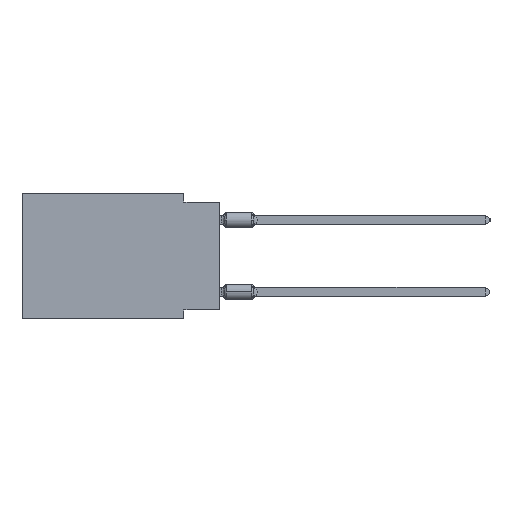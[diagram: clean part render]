
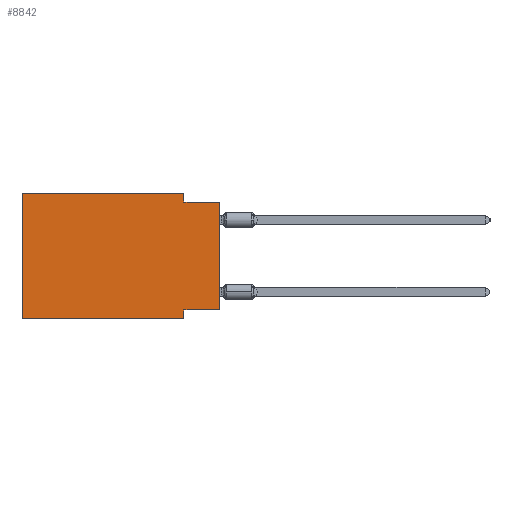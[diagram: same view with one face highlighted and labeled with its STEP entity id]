
A CAD part, left-side view. The second image highlights one B-rep face of the part: STEP entity #8842.
In plain terms, the highlighted planar face has unit normal (-1, 0, 0).
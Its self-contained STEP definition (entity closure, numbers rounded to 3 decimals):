
#359 = CARTESIAN_POINT ( 'NONE',  ( 0., 2.54, -8.89 ) ) ;
#743 = ORIENTED_EDGE ( 'NONE', *, *, #14845, .T. ) ;
#1000 = EDGE_CURVE ( 'NONE', #20234, #16087, #9139, .T. ) ;
#1103 = VECTOR ( 'NONE', #6230, 1000. ) ;
#1387 = EDGE_CURVE ( 'NONE', #20954, #15515, #6938, .T. ) ;
#1452 = DIRECTION ( 'NONE',  ( 0., -1., 0. ) ) ;
#2426 = CARTESIAN_POINT ( 'NONE',  ( 0., 13.97, -8.89 ) ) ;
#2891 = DIRECTION ( 'NONE',  ( 0., -1., 0. ) ) ;
#3227 = LINE ( 'NONE', #7388, #23684 ) ;
#3549 = CARTESIAN_POINT ( 'NONE',  ( 0., 0., -8.255 ) ) ;
#3810 = CARTESIAN_POINT ( 'NONE',  ( 0., 13.97, -8.89 ) ) ;
#3940 = CARTESIAN_POINT ( 'NONE',  ( 0., 13.97, 0. ) ) ;
#4109 = AXIS2_PLACEMENT_3D ( 'NONE', #7178, #11106, #23124 ) ;
#4303 = EDGE_LOOP ( 'NONE', ( #743, #24543, #21683, #19133, #11084, #18147, #22520, #16724 ) ) ;
#4856 = VECTOR ( 'NONE', #24507, 1000. ) ;
#5414 = CARTESIAN_POINT ( 'NONE',  ( 0., 2.54, -0.635 ) ) ;
#6230 = DIRECTION ( 'NONE',  ( 0., 0., -1. ) ) ;
#6813 = EDGE_CURVE ( 'NONE', #19035, #24148, #3227, .T. ) ;
#6938 = LINE ( 'NONE', #9159, #22282 ) ;
#7154 = EDGE_CURVE ( 'NONE', #15515, #20234, #12835, .T. ) ;
#7178 = CARTESIAN_POINT ( 'NONE',  ( 0., 13.97, 0. ) ) ;
#7388 = CARTESIAN_POINT ( 'NONE',  ( 0., 0., -8.255 ) ) ;
#7680 = CARTESIAN_POINT ( 'NONE',  ( 0., 0., 0. ) ) ;
#7709 = CARTESIAN_POINT ( 'NONE',  ( 0., 2.54, -8.255 ) ) ;
#8466 = CARTESIAN_POINT ( 'NONE',  ( 0., 2.54, -8.89 ) ) ;
#8629 = CARTESIAN_POINT ( 'NONE',  ( 0., 0., -0.635 ) ) ;
#8842 = ADVANCED_FACE ( 'NONE', ( #15046 ), #13058, .F. ) ;
#9139 = LINE ( 'NONE', #8629, #20208 ) ;
#9159 = CARTESIAN_POINT ( 'NONE',  ( 0., 13.97, 0. ) ) ;
#10782 = VERTEX_POINT ( 'NONE', #8466 ) ;
#11084 = ORIENTED_EDGE ( 'NONE', *, *, #15676, .F. ) ;
#11106 = DIRECTION ( 'NONE',  ( 1., 0., 0. ) ) ;
#12835 = LINE ( 'NONE', #16909, #16623 ) ;
#13058 = PLANE ( 'NONE',  #4109 ) ;
#13239 = VERTEX_POINT ( 'NONE', #3810 ) ;
#14677 = DIRECTION ( 'NONE',  ( 0., 0., -1. ) ) ;
#14845 = EDGE_CURVE ( 'NONE', #19035, #16087, #15930, .T. ) ;
#15046 = FACE_OUTER_BOUND ( 'NONE', #4303, .T. ) ;
#15515 = VERTEX_POINT ( 'NONE', #25122 ) ;
#15676 = EDGE_CURVE ( 'NONE', #13239, #20954, #18059, .T. ) ;
#15930 = LINE ( 'NONE', #7680, #24340 ) ;
#16087 = VERTEX_POINT ( 'NONE', #18026 ) ;
#16623 = VECTOR ( 'NONE', #14677, 1000. ) ;
#16724 = ORIENTED_EDGE ( 'NONE', *, *, #6813, .F. ) ;
#16909 = CARTESIAN_POINT ( 'NONE',  ( 0., 2.54, 0. ) ) ;
#18026 = CARTESIAN_POINT ( 'NONE',  ( 0., 0., -0.635 ) ) ;
#18059 = LINE ( 'NONE', #3940, #23543 ) ;
#18147 = ORIENTED_EDGE ( 'NONE', *, *, #19003, .T. ) ;
#19003 = EDGE_CURVE ( 'NONE', #13239, #10782, #20319, .T. ) ;
#19035 = VERTEX_POINT ( 'NONE', #3549 ) ;
#19133 = ORIENTED_EDGE ( 'NONE', *, *, #1387, .F. ) ;
#19429 = DIRECTION ( 'NONE',  ( 0., 1., 0. ) ) ;
#19877 = DIRECTION ( 'NONE',  ( 0., 0., 1. ) ) ;
#20080 = LINE ( 'NONE', #359, #1103 ) ;
#20208 = VECTOR ( 'NONE', #2891, 1000. ) ;
#20234 = VERTEX_POINT ( 'NONE', #5414 ) ;
#20319 = LINE ( 'NONE', #2426, #4856 ) ;
#20954 = VERTEX_POINT ( 'NONE', #21593 ) ;
#21593 = CARTESIAN_POINT ( 'NONE',  ( 0., 13.97, 0. ) ) ;
#21683 = ORIENTED_EDGE ( 'NONE', *, *, #7154, .F. ) ;
#21850 = EDGE_CURVE ( 'NONE', #24148, #10782, #20080, .T. ) ;
#22282 = VECTOR ( 'NONE', #1452, 1000. ) ;
#22520 = ORIENTED_EDGE ( 'NONE', *, *, #21850, .F. ) ;
#23124 = DIRECTION ( 'NONE',  ( 0., 0., -1. ) ) ;
#23543 = VECTOR ( 'NONE', #19877, 1000. ) ;
#23684 = VECTOR ( 'NONE', #19429, 1000. ) ;
#23885 = DIRECTION ( 'NONE',  ( 0., 0., 1. ) ) ;
#24148 = VERTEX_POINT ( 'NONE', #7709 ) ;
#24340 = VECTOR ( 'NONE', #23885, 1000. ) ;
#24507 = DIRECTION ( 'NONE',  ( 0., -1., 0. ) ) ;
#24543 = ORIENTED_EDGE ( 'NONE', *, *, #1000, .F. ) ;
#25122 = CARTESIAN_POINT ( 'NONE',  ( 0., 2.54, 0. ) ) ;
